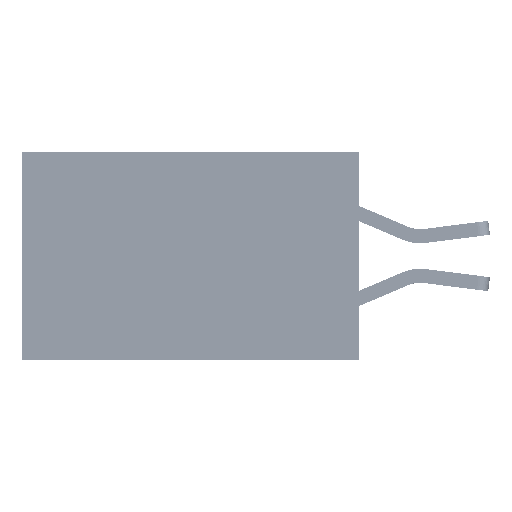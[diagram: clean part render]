
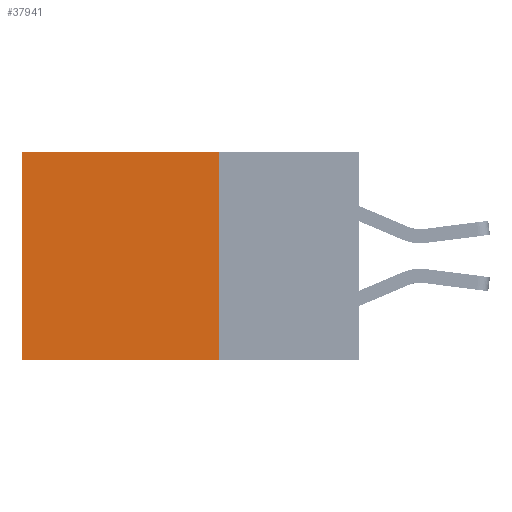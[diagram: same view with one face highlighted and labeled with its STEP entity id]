
A CAD part, left-side view. The second image highlights one B-rep face of the part: STEP entity #37941.
In plain terms, the highlighted planar face has unit normal (-1, 0, 0).
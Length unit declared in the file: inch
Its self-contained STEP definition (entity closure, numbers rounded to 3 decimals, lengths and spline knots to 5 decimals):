
#234 = DIRECTION ( 'NONE',  ( 0., 0., -1. ) ) ;
#463 = PLANE ( 'NONE',  #35376 ) ;
#1422 = ORIENTED_EDGE ( 'NONE', *, *, #14797, .F. ) ;
#3856 = LINE ( 'NONE', #32450, #22775 ) ;
#4153 = LINE ( 'NONE', #28815, #24329 ) ;
#5028 = VERTEX_POINT ( 'NONE', #23249 ) ;
#6980 = LINE ( 'NONE', #51332, #27058 ) ;
#7623 = VERTEX_POINT ( 'NONE', #8193 ) ;
#8193 = CARTESIAN_POINT ( 'NONE',  ( 0.2875, 0.25, -0.37 ) ) ;
#8701 = CARTESIAN_POINT ( 'NONE',  ( 0.2875, 0.6, 0. ) ) ;
#10270 = EDGE_CURVE ( 'NONE', #7623, #5028, #6980, .T. ) ;
#11527 = VECTOR ( 'NONE', #17707, 39.37008 ) ;
#14323 = EDGE_LOOP ( 'NONE', ( #50657, #28272, #1422, #41275 ) ) ;
#14797 = EDGE_CURVE ( 'NONE', #16447, #7623, #4153, .T. ) ;
#16447 = VERTEX_POINT ( 'NONE', #39736 ) ;
#16751 = DIRECTION ( 'NONE',  ( 0., 0., -1. ) ) ;
#17538 = CARTESIAN_POINT ( 'NONE',  ( 0.2875, 0.25, 0. ) ) ;
#17707 = DIRECTION ( 'NONE',  ( 0., 1., 0. ) ) ;
#22775 = VECTOR ( 'NONE', #234, 39.37008 ) ;
#23249 = CARTESIAN_POINT ( 'NONE',  ( 0.2875, 0.6, -0.37 ) ) ;
#23444 = VERTEX_POINT ( 'NONE', #8701 ) ;
#24329 = VECTOR ( 'NONE', #36890, 39.37008 ) ;
#24627 = CARTESIAN_POINT ( 'NONE',  ( 0.2875, 0.25, 0. ) ) ;
#26745 = FACE_OUTER_BOUND ( 'NONE', #14323, .T. ) ;
#26749 = EDGE_CURVE ( 'NONE', #23444, #5028, #3856, .T. ) ;
#27058 = VECTOR ( 'NONE', #47342, 39.37008 ) ;
#28272 = ORIENTED_EDGE ( 'NONE', *, *, #10270, .F. ) ;
#28815 = CARTESIAN_POINT ( 'NONE',  ( 0.2875, 0.25, 0. ) ) ;
#32450 = CARTESIAN_POINT ( 'NONE',  ( 0.2875, 0.6, 0. ) ) ;
#32913 = LINE ( 'NONE', #17538, #11527 ) ;
#33591 = EDGE_CURVE ( 'NONE', #16447, #23444, #32913, .T. ) ;
#35376 = AXIS2_PLACEMENT_3D ( 'NONE', #24627, #40770, #16751 ) ;
#36890 = DIRECTION ( 'NONE',  ( 0., 0., -1. ) ) ;
#37941 = ADVANCED_FACE ( 'NONE', ( #26745 ), #463, .F. ) ;
#39736 = CARTESIAN_POINT ( 'NONE',  ( 0.2875, 0.25, 0. ) ) ;
#40770 = DIRECTION ( 'NONE',  ( 1., 0., 0. ) ) ;
#41275 = ORIENTED_EDGE ( 'NONE', *, *, #33591, .T. ) ;
#47342 = DIRECTION ( 'NONE',  ( 0., 1., 0. ) ) ;
#50657 = ORIENTED_EDGE ( 'NONE', *, *, #26749, .T. ) ;
#51332 = CARTESIAN_POINT ( 'NONE',  ( 0.2875, 0.25, -0.37 ) ) ;
